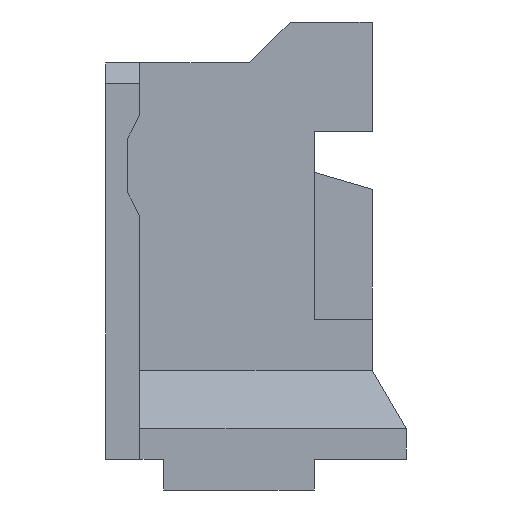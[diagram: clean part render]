
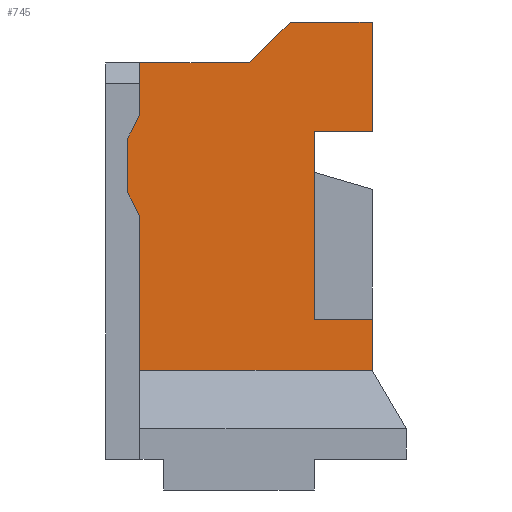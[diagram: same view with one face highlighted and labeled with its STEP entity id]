
A CAD part, left-side view. The second image highlights one B-rep face of the part: STEP entity #745.
In plain terms, the highlighted planar face has unit normal (-1, 0, 0).
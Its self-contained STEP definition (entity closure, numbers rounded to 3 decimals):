
#5 = EDGE_CURVE ( 'NONE', #268, #2809, #2136, .T. ) ;
#18 = ORIENTED_EDGE ( 'NONE', *, *, #1654, .F. ) ;
#52 = CARTESIAN_POINT ( 'NONE',  ( -1.25, 1.1, -0.75 ) ) ;
#141 = CARTESIAN_POINT ( 'NONE',  ( -1.25, 1.1, -0.75 ) ) ;
#175 = LINE ( 'NONE', #2709, #2223 ) ;
#201 = EDGE_CURVE ( 'NONE', #1115, #2662, #494, .T. ) ;
#217 = EDGE_CURVE ( 'NONE', #2470, #2175, #1072, .T. ) ;
#225 = DIRECTION ( 'NONE',  ( 0., 0., -1. ) ) ;
#268 = VERTEX_POINT ( 'NONE', #558 ) ;
#271 = ORIENTED_EDGE ( 'NONE', *, *, #5, .F. ) ;
#304 = CARTESIAN_POINT ( 'NONE',  ( -1.25, 1.275, -2.25 ) ) ;
#337 = DIRECTION ( 'NONE',  ( 0., -1., 0. ) ) ;
#348 = CARTESIAN_POINT ( 'NONE',  ( -1.25, 1.1, 0. ) ) ;
#363 = DIRECTION ( 'NONE',  ( 0., -0.707, 0.707 ) ) ;
#380 = DIRECTION ( 'NONE',  ( 0., 1., 0. ) ) ;
#412 = CARTESIAN_POINT ( 'NONE',  ( -1.25, -0.5, 0. ) ) ;
#447 = VECTOR ( 'NONE', #380, 1000. ) ;
#453 = ORIENTED_EDGE ( 'NONE', *, *, #2497, .F. ) ;
#475 = LINE ( 'NONE', #412, #2491 ) ;
#494 = LINE ( 'NONE', #348, #2166 ) ;
#530 = EDGE_CURVE ( 'NONE', #691, #2451, #1109, .T. ) ;
#538 = CARTESIAN_POINT ( 'NONE',  ( -1.25, 1.1, 0. ) ) ;
#558 = CARTESIAN_POINT ( 'NONE',  ( -1.25, -1.1, 0.6 ) ) ;
#621 = ORIENTED_EDGE ( 'NONE', *, *, #1362, .F. ) ;
#626 = CARTESIAN_POINT ( 'NONE',  ( -1.25, -2.3, 0.6 ) ) ;
#628 = PLANE ( 'NONE',  #2417 ) ;
#641 = DIRECTION ( 'NONE',  ( 1., 0., 0. ) ) ;
#691 = VERTEX_POINT ( 'NONE', #2776 ) ;
#698 = VECTOR ( 'NONE', #2825, 1000. ) ;
#742 = DIRECTION ( 'NONE',  ( 0., 0., 1. ) ) ;
#745 = ADVANCED_FACE ( 'NONE', ( #1555 ), #628, .F. ) ;
#795 = VECTOR ( 'NONE', #2379, 1000. ) ;
#839 = CARTESIAN_POINT ( 'NONE',  ( -1.25, 1.1, -2.25 ) ) ;
#843 = CARTESIAN_POINT ( 'NONE',  ( -1.25, -1.45, -3.75 ) ) ;
#859 = DIRECTION ( 'NONE',  ( 0., 0., -1. ) ) ;
#899 = VECTOR ( 'NONE', #225, 1000. ) ;
#926 = VECTOR ( 'NONE', #1744, 1000. ) ;
#933 = ORIENTED_EDGE ( 'NONE', *, *, #1463, .F. ) ;
#961 = CARTESIAN_POINT ( 'NONE',  ( -1.25, -2.3, -3.75 ) ) ;
#971 = LINE ( 'NONE', #2179, #1414 ) ;
#996 = CARTESIAN_POINT ( 'NONE',  ( -1.25, -2.3, -1. ) ) ;
#1006 = VECTOR ( 'NONE', #1854, 1000. ) ;
#1013 = ORIENTED_EDGE ( 'NONE', *, *, #2011, .F. ) ;
#1072 = LINE ( 'NONE', #141, #1006 ) ;
#1109 = LINE ( 'NONE', #2648, #795 ) ;
#1113 = EDGE_CURVE ( 'NONE', #1851, #2470, #2678, .T. ) ;
#1115 = VERTEX_POINT ( 'NONE', #538 ) ;
#1215 = CARTESIAN_POINT ( 'NONE',  ( -1.25, 1.275, -1.9 ) ) ;
#1274 = CARTESIAN_POINT ( 'NONE',  ( -1.25, 1.1, -5.8 ) ) ;
#1286 = DIRECTION ( 'NONE',  ( 0., -1., 0. ) ) ;
#1362 = EDGE_CURVE ( 'NONE', #2809, #1841, #2653, .T. ) ;
#1385 = DIRECTION ( 'NONE',  ( 0., 0., -1. ) ) ;
#1414 = VECTOR ( 'NONE', #1286, 1000. ) ;
#1420 = EDGE_CURVE ( 'NONE', #2471, #2322, #971, .T. ) ;
#1438 = ORIENTED_EDGE ( 'NONE', *, *, #201, .F. ) ;
#1463 = EDGE_CURVE ( 'NONE', #2451, #1851, #1787, .T. ) ;
#1470 = CARTESIAN_POINT ( 'NONE',  ( -1.25, -2.3, -1. ) ) ;
#1504 = CARTESIAN_POINT ( 'NONE',  ( -1.25, 1.1, -2.25 ) ) ;
#1520 = ORIENTED_EDGE ( 'NONE', *, *, #2783, .F. ) ;
#1540 = LINE ( 'NONE', #1733, #926 ) ;
#1554 = VECTOR ( 'NONE', #2229, 1000. ) ;
#1555 = FACE_OUTER_BOUND ( 'NONE', #1599, .T. ) ;
#1599 = EDGE_LOOP ( 'NONE', ( #1013, #2439, #2335, #933, #2090, #1693, #1520, #1897, #18, #2814, #621, #271, #453, #1438 ) ) ;
#1601 = LINE ( 'NONE', #1470, #447 ) ;
#1654 = EDGE_CURVE ( 'NONE', #2155, #2471, #175, .T. ) ;
#1680 = DIRECTION ( 'NONE',  ( 0., 0., 1. ) ) ;
#1693 = ORIENTED_EDGE ( 'NONE', *, *, #2060, .F. ) ;
#1710 = DIRECTION ( 'NONE',  ( 0., 0., -1. ) ) ;
#1722 = CARTESIAN_POINT ( 'NONE',  ( -1.25, -2.3, -4.5 ) ) ;
#1723 = CARTESIAN_POINT ( 'NONE',  ( -1.25, 0., 0. ) ) ;
#1733 = CARTESIAN_POINT ( 'NONE',  ( -1.25, -3., -4.5 ) ) ;
#1742 = CARTESIAN_POINT ( 'NONE',  ( -1.25, -2.3, -1.85 ) ) ;
#1744 = DIRECTION ( 'NONE',  ( 0., 1., 0. ) ) ;
#1749 = CARTESIAN_POINT ( 'NONE',  ( -1.25, -2.3, 0.6 ) ) ;
#1787 = LINE ( 'NONE', #839, #698 ) ;
#1841 = VERTEX_POINT ( 'NONE', #996 ) ;
#1843 = LINE ( 'NONE', #1742, #2420 ) ;
#1851 = VERTEX_POINT ( 'NONE', #1215 ) ;
#1854 = DIRECTION ( 'NONE',  ( 0., -0.447, 0.894 ) ) ;
#1897 = ORIENTED_EDGE ( 'NONE', *, *, #1420, .F. ) ;
#1983 = VECTOR ( 'NONE', #1680, 1000. ) ;
#2007 = EDGE_CURVE ( 'NONE', #1841, #2155, #1601, .T. ) ;
#2011 = EDGE_CURVE ( 'NONE', #2175, #1115, #2428, .T. ) ;
#2013 = CARTESIAN_POINT ( 'NONE',  ( -1.25, -1.1, 0.6 ) ) ;
#2060 = EDGE_CURVE ( 'NONE', #2108, #691, #1540, .T. ) ;
#2089 = CARTESIAN_POINT ( 'NONE',  ( -1.25, 1.275, -1.1 ) ) ;
#2090 = ORIENTED_EDGE ( 'NONE', *, *, #530, .F. ) ;
#2108 = VERTEX_POINT ( 'NONE', #1722 ) ;
#2125 = CARTESIAN_POINT ( 'NONE',  ( -1.25, -0.5, 0. ) ) ;
#2136 = LINE ( 'NONE', #2013, #1554 ) ;
#2155 = VERTEX_POINT ( 'NONE', #2443 ) ;
#2166 = VECTOR ( 'NONE', #337, 1000. ) ;
#2175 = VERTEX_POINT ( 'NONE', #52 ) ;
#2179 = CARTESIAN_POINT ( 'NONE',  ( -1.25, 3.057, -3.75 ) ) ;
#2223 = VECTOR ( 'NONE', #1385, 1000. ) ;
#2229 = DIRECTION ( 'NONE',  ( 0., -1., 0. ) ) ;
#2322 = VERTEX_POINT ( 'NONE', #961 ) ;
#2335 = ORIENTED_EDGE ( 'NONE', *, *, #1113, .F. ) ;
#2379 = DIRECTION ( 'NONE',  ( 0., 0., 1. ) ) ;
#2405 = VECTOR ( 'NONE', #742, 1000. ) ;
#2417 = AXIS2_PLACEMENT_3D ( 'NONE', #1723, #641, #859 ) ;
#2420 = VECTOR ( 'NONE', #1710, 1000. ) ;
#2428 = LINE ( 'NONE', #1274, #1983 ) ;
#2439 = ORIENTED_EDGE ( 'NONE', *, *, #217, .F. ) ;
#2443 = CARTESIAN_POINT ( 'NONE',  ( -1.25, -1.45, -1. ) ) ;
#2451 = VERTEX_POINT ( 'NONE', #1504 ) ;
#2470 = VERTEX_POINT ( 'NONE', #2089 ) ;
#2471 = VERTEX_POINT ( 'NONE', #843 ) ;
#2491 = VECTOR ( 'NONE', #363, 1000. ) ;
#2497 = EDGE_CURVE ( 'NONE', #2662, #268, #475, .T. ) ;
#2648 = CARTESIAN_POINT ( 'NONE',  ( -1.25, 1.1, -5.8 ) ) ;
#2653 = LINE ( 'NONE', #1749, #899 ) ;
#2662 = VERTEX_POINT ( 'NONE', #2125 ) ;
#2678 = LINE ( 'NONE', #304, #2405 ) ;
#2709 = CARTESIAN_POINT ( 'NONE',  ( -1.25, -1.45, -1. ) ) ;
#2776 = CARTESIAN_POINT ( 'NONE',  ( -1.25, 1.1, -4.5 ) ) ;
#2783 = EDGE_CURVE ( 'NONE', #2322, #2108, #1843, .T. ) ;
#2809 = VERTEX_POINT ( 'NONE', #626 ) ;
#2814 = ORIENTED_EDGE ( 'NONE', *, *, #2007, .F. ) ;
#2825 = DIRECTION ( 'NONE',  ( 0., 0.447, 0.894 ) ) ;
